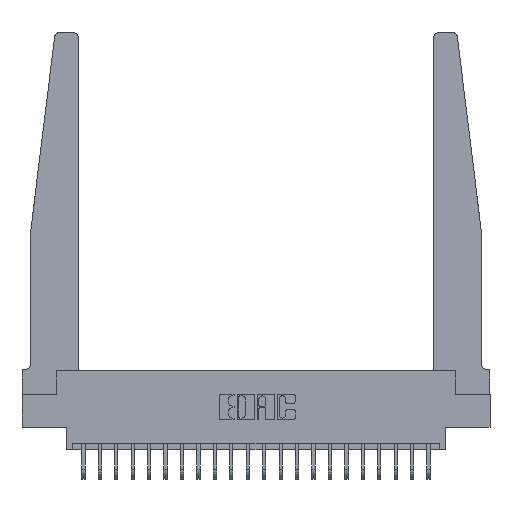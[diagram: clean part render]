
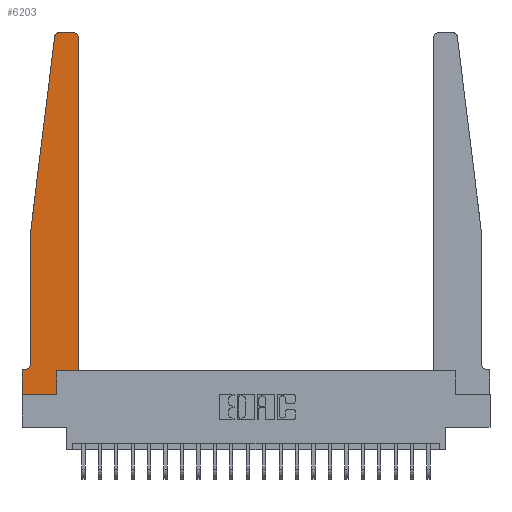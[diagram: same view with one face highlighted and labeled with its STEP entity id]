
A CAD part, top view. The second image highlights one B-rep face of the part: STEP entity #6203.
In plain terms, the highlighted planar face has unit normal (0, 0, 1).
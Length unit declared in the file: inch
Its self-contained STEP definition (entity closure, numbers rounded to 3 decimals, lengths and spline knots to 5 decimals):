
#373 = LINE ( 'NONE', #15421, #23095 ) ;
#517 = DIRECTION ( 'NONE',  ( 1., 0., 0. ) ) ;
#822 = VERTEX_POINT ( 'NONE', #19955 ) ;
#888 = ORIENTED_EDGE ( 'NONE', *, *, #22904, .T. ) ;
#1113 = EDGE_CURVE ( 'NONE', #21124, #19319, #14142, .T. ) ;
#1560 = CARTESIAN_POINT ( 'NONE',  ( 0.065, 1.25, 0.37 ) ) ;
#2329 = EDGE_CURVE ( 'NONE', #23915, #24015, #18194, .T. ) ;
#2339 = VECTOR ( 'NONE', #10490, 39.37008 ) ;
#2842 = LINE ( 'NONE', #6505, #19549 ) ;
#3591 = AXIS2_PLACEMENT_3D ( 'NONE', #20179, #4864, #22017 ) ;
#4367 = ORIENTED_EDGE ( 'NONE', *, *, #2329, .T. ) ;
#4509 = LINE ( 'NONE', #11981, #20199 ) ;
#4627 = EDGE_CURVE ( 'NONE', #24015, #9770, #9283, .T. ) ;
#4864 = DIRECTION ( 'NONE',  ( 0., 0., 1. ) ) ;
#5033 = VECTOR ( 'NONE', #17793, 39.37008 ) ;
#5391 = DIRECTION ( 'NONE',  ( 0., 0., -1. ) ) ;
#5524 = EDGE_CURVE ( 'NONE', #11269, #822, #373, .T. ) ;
#5924 = CARTESIAN_POINT ( 'NONE',  ( 0.425, 0.18, 0.37 ) ) ;
#6203 = ADVANCED_FACE ( 'NONE', ( #23833 ), #16482, .T. ) ;
#6293 = CARTESIAN_POINT ( 'NONE',  ( 0.2605, 0.18, 0.37 ) ) ;
#6336 = ORIENTED_EDGE ( 'NONE', *, *, #22178, .T. ) ;
#6433 = EDGE_CURVE ( 'NONE', #22782, #11269, #14545, .T. ) ;
#6457 = ORIENTED_EDGE ( 'NONE', *, *, #1113, .T. ) ;
#6505 = CARTESIAN_POINT ( 'NONE',  ( 0.425, 0.18, 0.37 ) ) ;
#6540 = VERTEX_POINT ( 'NONE', #17797 ) ;
#6795 = ORIENTED_EDGE ( 'NONE', *, *, #4627, .T. ) ;
#6901 = LINE ( 'NONE', #21837, #18401 ) ;
#7101 = AXIS2_PLACEMENT_3D ( 'NONE', #11264, #5391, #9182 ) ;
#7314 = EDGE_CURVE ( 'NONE', #20991, #21124, #10990, .T. ) ;
#7439 = ORIENTED_EDGE ( 'NONE', *, *, #12019, .T. ) ;
#7872 = EDGE_LOOP ( 'NONE', ( #20516, #7439, #4367, #6795, #888, #20019, #6457, #18241, #6336, #18850, #23189, #8283 ) ) ;
#8283 = ORIENTED_EDGE ( 'NONE', *, *, #6433, .T. ) ;
#9182 = DIRECTION ( 'NONE',  ( -1., 0., 0. ) ) ;
#9283 = LINE ( 'NONE', #20670, #19570 ) ;
#9315 = DIRECTION ( 'NONE',  ( -1., 0., 0. ) ) ;
#9709 = CARTESIAN_POINT ( 'NONE',  ( 0.395, 2.75, 0.37 ) ) ;
#9770 = VERTEX_POINT ( 'NONE', #14139 ) ;
#9836 = CIRCLE ( 'NONE', #7101, 0.05 ) ;
#9990 = CARTESIAN_POINT ( 'NONE',  ( 0., 0., 0.37 ) ) ;
#10059 = CARTESIAN_POINT ( 'NONE',  ( 0.065, 1.25, 0.37 ) ) ;
#10490 = DIRECTION ( 'NONE',  ( -0.122, -0.992, 0. ) ) ;
#10658 = DIRECTION ( 'NONE',  ( 1., 0., 0. ) ) ;
#10866 = DIRECTION ( 'NONE',  ( -1., 0., 0. ) ) ;
#10990 = LINE ( 'NONE', #19931, #20456 ) ;
#11245 = VERTEX_POINT ( 'NONE', #5924 ) ;
#11264 = CARTESIAN_POINT ( 'NONE',  ( 0.015, 0.2375, 0.37 ) ) ;
#11269 = VERTEX_POINT ( 'NONE', #9709 ) ;
#11830 = CARTESIAN_POINT ( 'NONE',  ( 0.395, 2.72, 0.37 ) ) ;
#11981 = CARTESIAN_POINT ( 'NONE',  ( 0., 0., 0.37 ) ) ;
#12019 = EDGE_CURVE ( 'NONE', #822, #23915, #19213, .T. ) ;
#12164 = LINE ( 'NONE', #6293, #14116 ) ;
#12186 = CARTESIAN_POINT ( 'NONE',  ( 0., 0., 0.37 ) ) ;
#12368 = CARTESIAN_POINT ( 'NONE',  ( 0.27653, 2.72, 0.37 ) ) ;
#12502 = CARTESIAN_POINT ( 'NONE',  ( 0.425, 2.72, 0.37 ) ) ;
#13081 = DIRECTION ( 'NONE',  ( 0., -1., 0. ) ) ;
#13376 = AXIS2_PLACEMENT_3D ( 'NONE', #11830, #14384, #16214 ) ;
#14116 = VECTOR ( 'NONE', #19637, 39.37008 ) ;
#14139 = CARTESIAN_POINT ( 'NONE',  ( 0.065, 0.2375, 0.37 ) ) ;
#14142 = LINE ( 'NONE', #12186, #5033 ) ;
#14384 = DIRECTION ( 'NONE',  ( 0., 0., 1. ) ) ;
#14545 = CIRCLE ( 'NONE', #13376, 0.03 ) ;
#15108 = EDGE_CURVE ( 'NONE', #19319, #22618, #4509, .T. ) ;
#15421 = CARTESIAN_POINT ( 'NONE',  ( 0.25, 2.75, 0.37 ) ) ;
#16214 = DIRECTION ( 'NONE',  ( 1., 0., 0. ) ) ;
#16482 = PLANE ( 'NONE',  #3591 ) ;
#17793 = DIRECTION ( 'NONE',  ( 0., -1., 0. ) ) ;
#17797 = CARTESIAN_POINT ( 'NONE',  ( 0.2605, 0.18, 0.37 ) ) ;
#18194 = LINE ( 'NONE', #1560, #2339 ) ;
#18241 = ORIENTED_EDGE ( 'NONE', *, *, #15108, .T. ) ;
#18387 = DIRECTION ( 'NONE',  ( 0., 1., 0. ) ) ;
#18401 = VECTOR ( 'NONE', #18387, 39.37008 ) ;
#18850 = ORIENTED_EDGE ( 'NONE', *, *, #21202, .T. ) ;
#18872 = CARTESIAN_POINT ( 'NONE',  ( 0., 0.1875, 0.37 ) ) ;
#19213 = CIRCLE ( 'NONE', #20780, 0.03 ) ;
#19319 = VERTEX_POINT ( 'NONE', #9990 ) ;
#19448 = DIRECTION ( 'NONE',  ( 1., 0., 0. ) ) ;
#19549 = VECTOR ( 'NONE', #517, 39.37008 ) ;
#19570 = VECTOR ( 'NONE', #13081, 39.37008 ) ;
#19637 = DIRECTION ( 'NONE',  ( 0., 1., 0. ) ) ;
#19734 = CARTESIAN_POINT ( 'NONE',  ( 0.24675, 2.72367, 0.37 ) ) ;
#19931 = CARTESIAN_POINT ( 'NONE',  ( 0.065, 0.1875, 0.37 ) ) ;
#19955 = CARTESIAN_POINT ( 'NONE',  ( 0.27653, 2.75, 0.37 ) ) ;
#19962 = DIRECTION ( 'NONE',  ( 0., 0., 1. ) ) ;
#20019 = ORIENTED_EDGE ( 'NONE', *, *, #7314, .T. ) ;
#20128 = CARTESIAN_POINT ( 'NONE',  ( 0.015, 0.1875, 0.37 ) ) ;
#20179 = CARTESIAN_POINT ( 'NONE',  ( 0., 0.1875, 0.37 ) ) ;
#20199 = VECTOR ( 'NONE', #19448, 39.37008 ) ;
#20456 = VECTOR ( 'NONE', #10866, 39.37008 ) ;
#20516 = ORIENTED_EDGE ( 'NONE', *, *, #5524, .T. ) ;
#20670 = CARTESIAN_POINT ( 'NONE',  ( 0.065, 1.25, 0.37 ) ) ;
#20780 = AXIS2_PLACEMENT_3D ( 'NONE', #12368, #19962, #10658 ) ;
#20991 = VERTEX_POINT ( 'NONE', #20128 ) ;
#21124 = VERTEX_POINT ( 'NONE', #18872 ) ;
#21202 = EDGE_CURVE ( 'NONE', #6540, #11245, #2842, .T. ) ;
#21440 = CARTESIAN_POINT ( 'NONE',  ( 0.2605, 0., 0.37 ) ) ;
#21837 = CARTESIAN_POINT ( 'NONE',  ( 0.425, 0.18, 0.37 ) ) ;
#22017 = DIRECTION ( 'NONE',  ( 1., 0., 0. ) ) ;
#22178 = EDGE_CURVE ( 'NONE', #22618, #6540, #12164, .T. ) ;
#22618 = VERTEX_POINT ( 'NONE', #21440 ) ;
#22782 = VERTEX_POINT ( 'NONE', #12502 ) ;
#22904 = EDGE_CURVE ( 'NONE', #9770, #20991, #9836, .T. ) ;
#23095 = VECTOR ( 'NONE', #9315, 39.37008 ) ;
#23189 = ORIENTED_EDGE ( 'NONE', *, *, #23789, .T. ) ;
#23789 = EDGE_CURVE ( 'NONE', #11245, #22782, #6901, .T. ) ;
#23833 = FACE_OUTER_BOUND ( 'NONE', #7872, .T. ) ;
#23915 = VERTEX_POINT ( 'NONE', #19734 ) ;
#24015 = VERTEX_POINT ( 'NONE', #10059 ) ;
